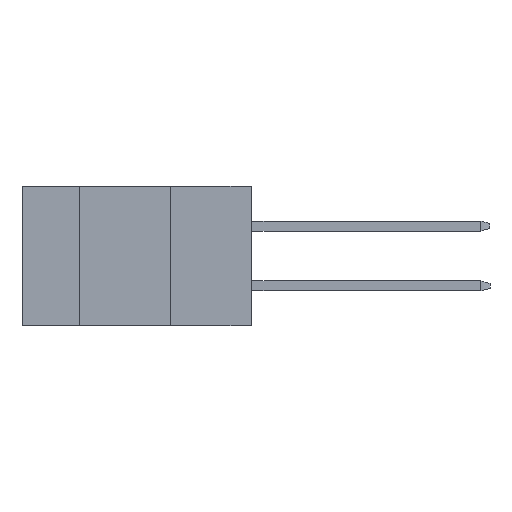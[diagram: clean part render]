
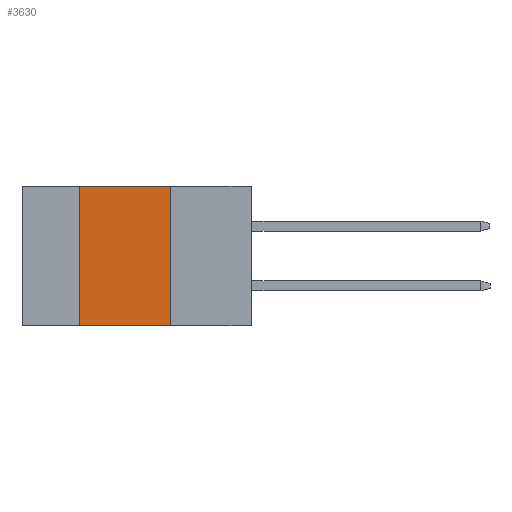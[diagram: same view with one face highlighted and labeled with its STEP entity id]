
A CAD part, left-side view. The second image highlights one B-rep face of the part: STEP entity #3630.
In plain terms, the highlighted planar face has unit normal (-1, 0, 0).
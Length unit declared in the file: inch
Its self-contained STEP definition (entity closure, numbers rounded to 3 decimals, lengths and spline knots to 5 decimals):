
#2197 = EDGE_CURVE ( 'NONE', #19226, #10531, #8863, .T. ) ;
#2359 = CARTESIAN_POINT ( 'NONE',  ( 0., 0.54, -0.437 ) ) ;
#2791 = VECTOR ( 'NONE', #13345, 39.37008 ) ;
#3068 = CARTESIAN_POINT ( 'NONE',  ( 0., 0.254, -0.437 ) ) ;
#3439 = CARTESIAN_POINT ( 'NONE',  ( 0., 0.54, 0. ) ) ;
#3630 = ADVANCED_FACE ( 'NONE', ( #15885 ), #14707, .F. ) ;
#3930 = VECTOR ( 'NONE', #8528, 39.37008 ) ;
#4117 = LINE ( 'NONE', #9811, #3930 ) ;
#4132 = DIRECTION ( 'NONE',  ( 1., 0., 0. ) ) ;
#4326 = DIRECTION ( 'NONE',  ( 0., 0., -1. ) ) ;
#5082 = AXIS2_PLACEMENT_3D ( 'NONE', #16084, #4132, #4326 ) ;
#5724 = VECTOR ( 'NONE', #16525, 39.37008 ) ;
#6455 = VECTOR ( 'NONE', #13669, 39.37008 ) ;
#6912 = ORIENTED_EDGE ( 'NONE', *, *, #2197, .F. ) ;
#6937 = ORIENTED_EDGE ( 'NONE', *, *, #9896, .T. ) ;
#7368 = CARTESIAN_POINT ( 'NONE',  ( 0., 0.54, -0.437 ) ) ;
#8528 = DIRECTION ( 'NONE',  ( 0., -1., 0. ) ) ;
#8863 = LINE ( 'NONE', #7368, #2791 ) ;
#9811 = CARTESIAN_POINT ( 'NONE',  ( 0., 0.72, 0. ) ) ;
#9896 = EDGE_CURVE ( 'NONE', #19226, #16710, #14858, .T. ) ;
#10531 = VERTEX_POINT ( 'NONE', #3439 ) ;
#11443 = EDGE_LOOP ( 'NONE', ( #16646, #15541, #6912, #6937 ) ) ;
#11831 = CARTESIAN_POINT ( 'NONE',  ( 0., 0.72, -0.437 ) ) ;
#13345 = DIRECTION ( 'NONE',  ( 0., 0., 1. ) ) ;
#13669 = DIRECTION ( 'NONE',  ( 0., -1., 0. ) ) ;
#14707 = PLANE ( 'NONE',  #5082 ) ;
#14766 = LINE ( 'NONE', #15048, #5724 ) ;
#14858 = LINE ( 'NONE', #11831, #6455 ) ;
#15048 = CARTESIAN_POINT ( 'NONE',  ( 0., 0.254, -0.437 ) ) ;
#15541 = ORIENTED_EDGE ( 'NONE', *, *, #18370, .F. ) ;
#15885 = FACE_OUTER_BOUND ( 'NONE', #11443, .T. ) ;
#16084 = CARTESIAN_POINT ( 'NONE',  ( 0., 0.72, 0. ) ) ;
#16268 = CARTESIAN_POINT ( 'NONE',  ( 0., 0.254, 0. ) ) ;
#16525 = DIRECTION ( 'NONE',  ( 0., 0., -1. ) ) ;
#16646 = ORIENTED_EDGE ( 'NONE', *, *, #17066, .F. ) ;
#16710 = VERTEX_POINT ( 'NONE', #3068 ) ;
#17066 = EDGE_CURVE ( 'NONE', #18473, #16710, #14766, .T. ) ;
#18370 = EDGE_CURVE ( 'NONE', #10531, #18473, #4117, .T. ) ;
#18473 = VERTEX_POINT ( 'NONE', #16268 ) ;
#19226 = VERTEX_POINT ( 'NONE', #2359 ) ;
